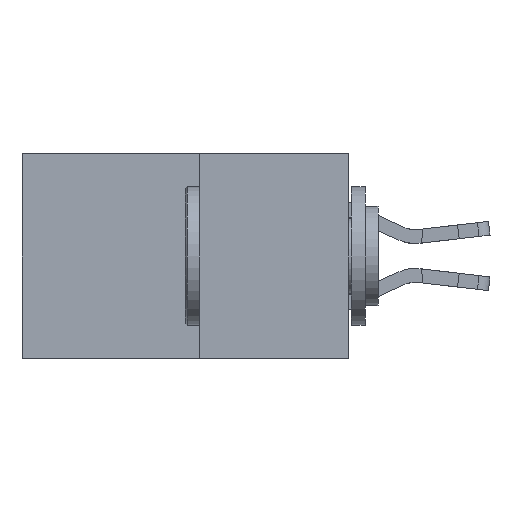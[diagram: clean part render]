
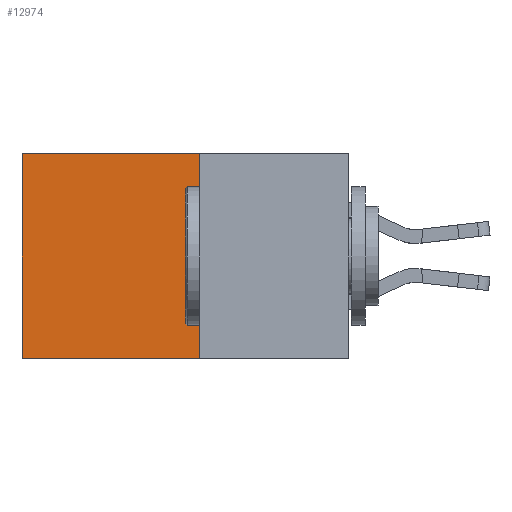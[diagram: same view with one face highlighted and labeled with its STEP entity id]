
A CAD part, left-side view. The second image highlights one B-rep face of the part: STEP entity #12974.
In plain terms, the highlighted planar face has unit normal (-1, 0, 0).
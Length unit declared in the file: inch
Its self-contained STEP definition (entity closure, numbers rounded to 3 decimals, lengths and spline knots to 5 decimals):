
#997 = LINE ( 'NONE', #5249, #20884 ) ;
#1306 = DIRECTION ( 'NONE',  ( 0., 0., -1. ) ) ;
#3095 = CARTESIAN_POINT ( 'NONE',  ( 0.277, 0.59, -0.37 ) ) ;
#3154 = VERTEX_POINT ( 'NONE', #3095 ) ;
#3256 = PLANE ( 'NONE',  #3673 ) ;
#3341 = DIRECTION ( 'NONE',  ( 1., 0., 0. ) ) ;
#3673 = AXIS2_PLACEMENT_3D ( 'NONE', #15044, #3341, #16970 ) ;
#4581 = VERTEX_POINT ( 'NONE', #10933 ) ;
#5032 = LINE ( 'NONE', #5152, #19780 ) ;
#5033 = CARTESIAN_POINT ( 'NONE',  ( 0.277, 0.59, 0. ) ) ;
#5152 = CARTESIAN_POINT ( 'NONE',  ( 0.277, 0.27, -0.37 ) ) ;
#5249 = CARTESIAN_POINT ( 'NONE',  ( 0.277, 0.27, -0.37 ) ) ;
#6302 = DIRECTION ( 'NONE',  ( 0., 1., 0. ) ) ;
#6715 = ORIENTED_EDGE ( 'NONE', *, *, #17683, .T. ) ;
#7139 = DIRECTION ( 'NONE',  ( 0., 0., -1. ) ) ;
#7242 = DIRECTION ( 'NONE',  ( 0., 1., 0. ) ) ;
#9011 = VECTOR ( 'NONE', #1306, 39.37008 ) ;
#9061 = ORIENTED_EDGE ( 'NONE', *, *, #17666, .F. ) ;
#9616 = LINE ( 'NONE', #11062, #9011 ) ;
#10764 = EDGE_CURVE ( 'NONE', #12917, #3154, #997, .T. ) ;
#10933 = CARTESIAN_POINT ( 'NONE',  ( 0.277, 0.27, 0. ) ) ;
#11062 = CARTESIAN_POINT ( 'NONE',  ( 0.277, 0.59, -0.37 ) ) ;
#12170 = LINE ( 'NONE', #23372, #21663 ) ;
#12917 = VERTEX_POINT ( 'NONE', #14885 ) ;
#12974 = ADVANCED_FACE ( 'NONE', ( #22744 ), #3256, .F. ) ;
#14885 = CARTESIAN_POINT ( 'NONE',  ( 0.277, 0.27, -0.37 ) ) ;
#15044 = CARTESIAN_POINT ( 'NONE',  ( 0.277, 0.27, -0.37 ) ) ;
#15578 = ORIENTED_EDGE ( 'NONE', *, *, #10764, .F. ) ;
#15595 = VERTEX_POINT ( 'NONE', #5033 ) ;
#16970 = DIRECTION ( 'NONE',  ( 0., 0., -1. ) ) ;
#17666 = EDGE_CURVE ( 'NONE', #4581, #12917, #5032, .T. ) ;
#17683 = EDGE_CURVE ( 'NONE', #15595, #3154, #9616, .T. ) ;
#19780 = VECTOR ( 'NONE', #7139, 39.37008 ) ;
#20610 = ORIENTED_EDGE ( 'NONE', *, *, #20841, .T. ) ;
#20841 = EDGE_CURVE ( 'NONE', #4581, #15595, #12170, .T. ) ;
#20884 = VECTOR ( 'NONE', #7242, 39.37008 ) ;
#21663 = VECTOR ( 'NONE', #6302, 39.37008 ) ;
#22744 = FACE_OUTER_BOUND ( 'NONE', #22874, .T. ) ;
#22874 = EDGE_LOOP ( 'NONE', ( #6715, #15578, #9061, #20610 ) ) ;
#23372 = CARTESIAN_POINT ( 'NONE',  ( 0.277, 0.27, 0. ) ) ;
